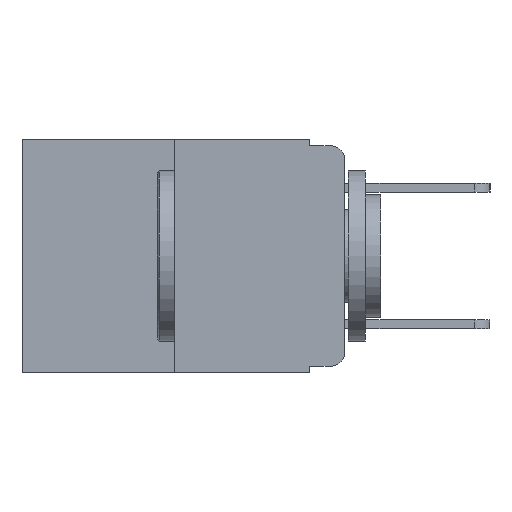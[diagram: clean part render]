
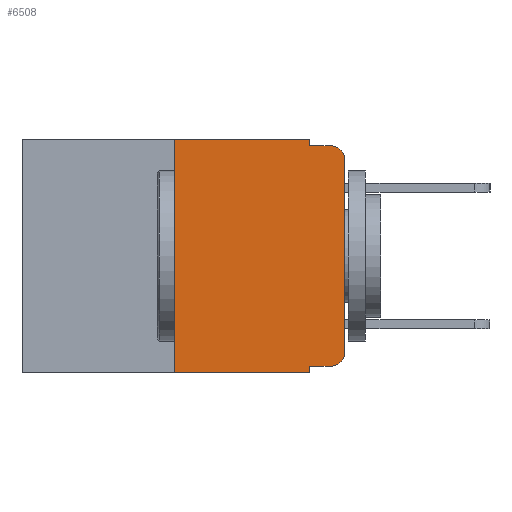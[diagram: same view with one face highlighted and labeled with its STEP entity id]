
A CAD part, left-side view. The second image highlights one B-rep face of the part: STEP entity #6508.
In plain terms, the highlighted planar face has unit normal (-1, 0, 0).
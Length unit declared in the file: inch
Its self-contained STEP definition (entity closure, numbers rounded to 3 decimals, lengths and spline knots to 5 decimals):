
#185 = ORIENTED_EDGE ( 'NONE', *, *, #2248, .T. ) ;
#255 = AXIS2_PLACEMENT_3D ( 'NONE', #3812, #10427, #4803 ) ;
#457 = VECTOR ( 'NONE', #692, 39.37008 ) ;
#692 = DIRECTION ( 'NONE',  ( 0., -1., 0. ) ) ;
#698 = DIRECTION ( 'NONE',  ( 0., 0., -1. ) ) ;
#781 = LINE ( 'NONE', #11823, #457 ) ;
#849 = LINE ( 'NONE', #6495, #3088 ) ;
#1100 = PLANE ( 'NONE',  #2070 ) ;
#1173 = VECTOR ( 'NONE', #5891, 39.37008 ) ;
#1283 = EDGE_CURVE ( 'NONE', #11813, #9318, #9069, .T. ) ;
#1292 = CARTESIAN_POINT ( 'NONE',  ( 0., 0.051, -0.01 ) ) ;
#1652 = ORIENTED_EDGE ( 'NONE', *, *, #11571, .T. ) ;
#2065 = CARTESIAN_POINT ( 'NONE',  ( 0., 0.473, 0. ) ) ;
#2070 = AXIS2_PLACEMENT_3D ( 'NONE', #2065, #8798, #3031 ) ;
#2248 = EDGE_CURVE ( 'NONE', #11368, #8133, #781, .T. ) ;
#2340 = CARTESIAN_POINT ( 'NONE',  ( 0., 0., 0. ) ) ;
#2461 = CARTESIAN_POINT ( 'NONE',  ( 0., 0.051, -0.01 ) ) ;
#2920 = CARTESIAN_POINT ( 'NONE',  ( 0., 0.051, 0. ) ) ;
#3031 = DIRECTION ( 'NONE',  ( 0., 0., -1. ) ) ;
#3088 = VECTOR ( 'NONE', #698, 39.37008 ) ;
#3195 = DIRECTION ( 'NONE',  ( 0., -1., 0. ) ) ;
#3210 = EDGE_CURVE ( 'NONE', #3340, #11813, #4515, .T. ) ;
#3340 = VERTEX_POINT ( 'NONE', #2920 ) ;
#3812 = CARTESIAN_POINT ( 'NONE',  ( 0., 0.02, -0.03 ) ) ;
#4126 = VECTOR ( 'NONE', #3195, 39.37008 ) ;
#4342 = LINE ( 'NONE', #10358, #1173 ) ;
#4347 = DIRECTION ( 'NONE',  ( 0., 0., 1. ) ) ;
#4392 = ORIENTED_EDGE ( 'NONE', *, *, #5828, .F. ) ;
#4399 = VERTEX_POINT ( 'NONE', #8432 ) ;
#4484 = ORIENTED_EDGE ( 'NONE', *, *, #9616, .T. ) ;
#4502 = EDGE_CURVE ( 'NONE', #11368, #8953, #4342, .T. ) ;
#4515 = LINE ( 'NONE', #5268, #9304 ) ;
#4668 = ORIENTED_EDGE ( 'NONE', *, *, #10428, .T. ) ;
#4789 = CIRCLE ( 'NONE', #11589, 0.02 ) ;
#4803 = DIRECTION ( 'NONE',  ( 0., 0., -1. ) ) ;
#4860 = CARTESIAN_POINT ( 'NONE',  ( 0., 0.25, 0. ) ) ;
#5023 = CARTESIAN_POINT ( 'NONE',  ( 0., 0.02, -0.313 ) ) ;
#5063 = ORIENTED_EDGE ( 'NONE', *, *, #7773, .T. ) ;
#5250 = LINE ( 'NONE', #2340, #7527 ) ;
#5268 = CARTESIAN_POINT ( 'NONE',  ( 0., 0.051, 0. ) ) ;
#5602 = VERTEX_POINT ( 'NONE', #10689 ) ;
#5828 = EDGE_CURVE ( 'NONE', #6541, #8133, #849, .T. ) ;
#5891 = DIRECTION ( 'NONE',  ( 0., 0., 1. ) ) ;
#5984 = DIRECTION ( 'NONE',  ( 0., 0., -1. ) ) ;
#6364 = DIRECTION ( 'NONE',  ( 0., -1., 0. ) ) ;
#6377 = CARTESIAN_POINT ( 'NONE',  ( 0., 0., -0.03 ) ) ;
#6495 = CARTESIAN_POINT ( 'NONE',  ( 0., 0.051, 0. ) ) ;
#6508 = ADVANCED_FACE ( 'NONE', ( #7934 ), #1100, .F. ) ;
#6541 = VERTEX_POINT ( 'NONE', #10636 ) ;
#6555 = VECTOR ( 'NONE', #6364, 39.37008 ) ;
#6632 = EDGE_CURVE ( 'NONE', #8953, #3340, #7338, .T. ) ;
#6677 = LINE ( 'NONE', #8978, #6983 ) ;
#6772 = VERTEX_POINT ( 'NONE', #6377 ) ;
#6914 = EDGE_LOOP ( 'NONE', ( #4668, #1652, #10548, #11376, #7748, #7900, #185, #4392, #5063, #4484 ) ) ;
#6983 = VECTOR ( 'NONE', #10712, 39.37008 ) ;
#7338 = LINE ( 'NONE', #8966, #4126 ) ;
#7527 = VECTOR ( 'NONE', #4347, 39.37008 ) ;
#7648 = CIRCLE ( 'NONE', #255, 0.02 ) ;
#7748 = ORIENTED_EDGE ( 'NONE', *, *, #6632, .F. ) ;
#7773 = EDGE_CURVE ( 'NONE', #6541, #4399, #6677, .T. ) ;
#7900 = ORIENTED_EDGE ( 'NONE', *, *, #4502, .F. ) ;
#7934 = FACE_OUTER_BOUND ( 'NONE', #6914, .T. ) ;
#8133 = VERTEX_POINT ( 'NONE', #10409 ) ;
#8432 = CARTESIAN_POINT ( 'NONE',  ( 0., 0.02, -0.333 ) ) ;
#8798 = DIRECTION ( 'NONE',  ( 1., 0., 0. ) ) ;
#8953 = VERTEX_POINT ( 'NONE', #4860 ) ;
#8966 = CARTESIAN_POINT ( 'NONE',  ( 0., 0.473, 0. ) ) ;
#8978 = CARTESIAN_POINT ( 'NONE',  ( 0., 0.051, -0.333 ) ) ;
#9069 = LINE ( 'NONE', #2461, #6555 ) ;
#9191 = CARTESIAN_POINT ( 'NONE',  ( 0., 0.02, -0.01 ) ) ;
#9304 = VECTOR ( 'NONE', #10138, 39.37008 ) ;
#9318 = VERTEX_POINT ( 'NONE', #9191 ) ;
#9616 = EDGE_CURVE ( 'NONE', #4399, #5602, #4789, .T. ) ;
#10138 = DIRECTION ( 'NONE',  ( 0., 0., -1. ) ) ;
#10358 = CARTESIAN_POINT ( 'NONE',  ( 0., 0.25, 0. ) ) ;
#10409 = CARTESIAN_POINT ( 'NONE',  ( 0., 0.051, -0.343 ) ) ;
#10427 = DIRECTION ( 'NONE',  ( -1., 0., 0. ) ) ;
#10428 = EDGE_CURVE ( 'NONE', #5602, #6772, #5250, .T. ) ;
#10548 = ORIENTED_EDGE ( 'NONE', *, *, #1283, .F. ) ;
#10636 = CARTESIAN_POINT ( 'NONE',  ( 0., 0.051, -0.333 ) ) ;
#10689 = CARTESIAN_POINT ( 'NONE',  ( 0., 0., -0.313 ) ) ;
#10712 = DIRECTION ( 'NONE',  ( 0., -1., 0. ) ) ;
#10950 = CARTESIAN_POINT ( 'NONE',  ( 0., 0.25, -0.343 ) ) ;
#11368 = VERTEX_POINT ( 'NONE', #10950 ) ;
#11376 = ORIENTED_EDGE ( 'NONE', *, *, #3210, .F. ) ;
#11464 = DIRECTION ( 'NONE',  ( -1., 0., 0. ) ) ;
#11571 = EDGE_CURVE ( 'NONE', #6772, #9318, #7648, .T. ) ;
#11589 = AXIS2_PLACEMENT_3D ( 'NONE', #5023, #11464, #5984 ) ;
#11813 = VERTEX_POINT ( 'NONE', #1292 ) ;
#11823 = CARTESIAN_POINT ( 'NONE',  ( 0., 0.473, -0.343 ) ) ;
